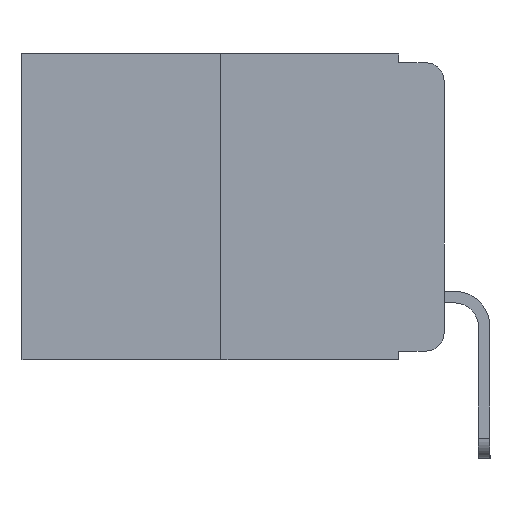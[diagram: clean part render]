
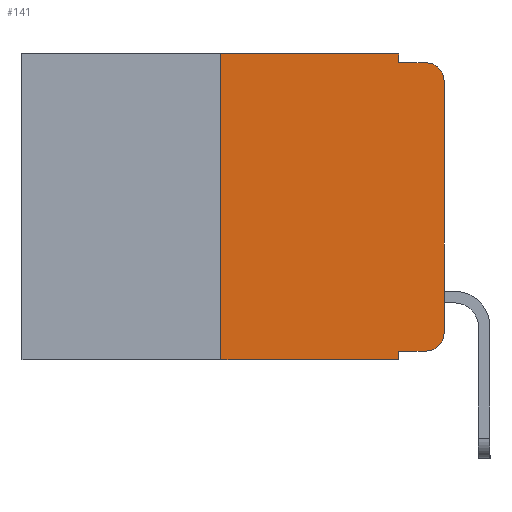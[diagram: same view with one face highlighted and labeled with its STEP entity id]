
A CAD part, left-side view. The second image highlights one B-rep face of the part: STEP entity #141.
In plain terms, the highlighted planar face has unit normal (-1, 0, 0).
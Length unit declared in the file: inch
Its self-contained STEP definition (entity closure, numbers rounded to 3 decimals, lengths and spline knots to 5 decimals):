
#25 = DIRECTION ( 'NONE',  ( 0., 0., 1. ) ) ;
#141 = ADVANCED_FACE ( 'NONE', ( #5684 ), #10027, .F. ) ;
#240 = EDGE_CURVE ( 'NONE', #4264, #10251, #3915, .T. ) ;
#488 = CARTESIAN_POINT ( 'NONE',  ( 0., 0.02, -0.03 ) ) ;
#715 = CARTESIAN_POINT ( 'NONE',  ( 0., 0.02, -0.01 ) ) ;
#745 = DIRECTION ( 'NONE',  ( 0., 0., -1. ) ) ;
#828 = DIRECTION ( 'NONE',  ( -1., 0., 0. ) ) ;
#872 = CARTESIAN_POINT ( 'NONE',  ( 0., 0.051, 0. ) ) ;
#1058 = VECTOR ( 'NONE', #2908, 39.37008 ) ;
#1182 = CARTESIAN_POINT ( 'NONE',  ( 0., 0.02, -0.333 ) ) ;
#1365 = EDGE_CURVE ( 'NONE', #10251, #9961, #12250, .T. ) ;
#1483 = VECTOR ( 'NONE', #25, 39.37008 ) ;
#1521 = VECTOR ( 'NONE', #1560, 39.37008 ) ;
#1560 = DIRECTION ( 'NONE',  ( 0., 0., 1. ) ) ;
#1778 = DIRECTION ( 'NONE',  ( -1., 0., 0. ) ) ;
#1791 = DIRECTION ( 'NONE',  ( 0., -1., 0. ) ) ;
#2551 = ORIENTED_EDGE ( 'NONE', *, *, #5349, .T. ) ;
#2644 = EDGE_CURVE ( 'NONE', #12869, #10065, #5430, .T. ) ;
#2698 = AXIS2_PLACEMENT_3D ( 'NONE', #488, #1778, #5899 ) ;
#2858 = LINE ( 'NONE', #7177, #7730 ) ;
#2908 = DIRECTION ( 'NONE',  ( 0., -1., 0. ) ) ;
#2915 = VERTEX_POINT ( 'NONE', #872 ) ;
#3318 = CARTESIAN_POINT ( 'NONE',  ( 0., 0., 0. ) ) ;
#3397 = EDGE_CURVE ( 'NONE', #5136, #4264, #13299, .T. ) ;
#3454 = ORIENTED_EDGE ( 'NONE', *, *, #7066, .F. ) ;
#3545 = EDGE_LOOP ( 'NONE', ( #9908, #2551, #11814, #5180, #7015, #3454, #7256, #12680, #9693, #5321 ) ) ;
#3559 = LINE ( 'NONE', #4491, #11255 ) ;
#3915 = CIRCLE ( 'NONE', #11914, 0.02 ) ;
#4149 = EDGE_CURVE ( 'NONE', #2915, #12869, #9555, .T. ) ;
#4264 = VERTEX_POINT ( 'NONE', #1182 ) ;
#4368 = CARTESIAN_POINT ( 'NONE',  ( 0., 0.051, -0.343 ) ) ;
#4491 = CARTESIAN_POINT ( 'NONE',  ( 0., 0.051, 0. ) ) ;
#4699 = VECTOR ( 'NONE', #11988, 39.37008 ) ;
#4989 = CIRCLE ( 'NONE', #2698, 0.02 ) ;
#5136 = VERTEX_POINT ( 'NONE', #11007 ) ;
#5180 = ORIENTED_EDGE ( 'NONE', *, *, #4149, .F. ) ;
#5321 = ORIENTED_EDGE ( 'NONE', *, *, #240, .T. ) ;
#5349 = EDGE_CURVE ( 'NONE', #9961, #10065, #4989, .T. ) ;
#5430 = LINE ( 'NONE', #11001, #4699 ) ;
#5605 = DIRECTION ( 'NONE',  ( 0., -1., 0. ) ) ;
#5684 = FACE_OUTER_BOUND ( 'NONE', #3545, .T. ) ;
#5819 = DIRECTION ( 'NONE',  ( 0., 0., -1. ) ) ;
#5899 = DIRECTION ( 'NONE',  ( 0., 0., -1. ) ) ;
#6280 = VERTEX_POINT ( 'NONE', #4368 ) ;
#6712 = VERTEX_POINT ( 'NONE', #10239 ) ;
#7015 = ORIENTED_EDGE ( 'NONE', *, *, #12361, .F. ) ;
#7066 = EDGE_CURVE ( 'NONE', #9452, #6712, #9349, .T. ) ;
#7177 = CARTESIAN_POINT ( 'NONE',  ( 0., 0.473, -0.343 ) ) ;
#7256 = ORIENTED_EDGE ( 'NONE', *, *, #11709, .T. ) ;
#7360 = CARTESIAN_POINT ( 'NONE',  ( 0., 0.051, 0. ) ) ;
#7667 = CARTESIAN_POINT ( 'NONE',  ( 0., 0.051, -0.333 ) ) ;
#7730 = VECTOR ( 'NONE', #1791, 39.37008 ) ;
#7891 = DIRECTION ( 'NONE',  ( 1., 0., 0. ) ) ;
#8069 = EDGE_CURVE ( 'NONE', #5136, #6280, #3559, .T. ) ;
#8197 = VECTOR ( 'NONE', #745, 39.37008 ) ;
#8271 = CARTESIAN_POINT ( 'NONE',  ( 0., 0.25, -0.343 ) ) ;
#8882 = CARTESIAN_POINT ( 'NONE',  ( 0., 0., -0.313 ) ) ;
#8958 = CARTESIAN_POINT ( 'NONE',  ( 0., 0.473, 0. ) ) ;
#9349 = LINE ( 'NONE', #13606, #1521 ) ;
#9452 = VERTEX_POINT ( 'NONE', #8271 ) ;
#9483 = LINE ( 'NONE', #9564, #1058 ) ;
#9555 = LINE ( 'NONE', #7360, #8197 ) ;
#9564 = CARTESIAN_POINT ( 'NONE',  ( 0., 0.473, 0. ) ) ;
#9693 = ORIENTED_EDGE ( 'NONE', *, *, #3397, .T. ) ;
#9908 = ORIENTED_EDGE ( 'NONE', *, *, #1365, .T. ) ;
#9961 = VERTEX_POINT ( 'NONE', #13721 ) ;
#10027 = PLANE ( 'NONE',  #12577 ) ;
#10065 = VERTEX_POINT ( 'NONE', #715 ) ;
#10103 = DIRECTION ( 'NONE',  ( 0., 0., -1. ) ) ;
#10239 = CARTESIAN_POINT ( 'NONE',  ( 0., 0.25, 0. ) ) ;
#10251 = VERTEX_POINT ( 'NONE', #8882 ) ;
#10439 = CARTESIAN_POINT ( 'NONE',  ( 0., 0.02, -0.313 ) ) ;
#11001 = CARTESIAN_POINT ( 'NONE',  ( 0., 0.051, -0.01 ) ) ;
#11007 = CARTESIAN_POINT ( 'NONE',  ( 0., 0.051, -0.333 ) ) ;
#11255 = VECTOR ( 'NONE', #5819, 39.37008 ) ;
#11574 = VECTOR ( 'NONE', #5605, 39.37008 ) ;
#11709 = EDGE_CURVE ( 'NONE', #9452, #6280, #2858, .T. ) ;
#11814 = ORIENTED_EDGE ( 'NONE', *, *, #2644, .F. ) ;
#11914 = AXIS2_PLACEMENT_3D ( 'NONE', #10439, #828, #13827 ) ;
#11988 = DIRECTION ( 'NONE',  ( 0., -1., 0. ) ) ;
#12250 = LINE ( 'NONE', #3318, #1483 ) ;
#12361 = EDGE_CURVE ( 'NONE', #6712, #2915, #9483, .T. ) ;
#12577 = AXIS2_PLACEMENT_3D ( 'NONE', #8958, #7891, #10103 ) ;
#12680 = ORIENTED_EDGE ( 'NONE', *, *, #8069, .F. ) ;
#12869 = VERTEX_POINT ( 'NONE', #14015 ) ;
#13299 = LINE ( 'NONE', #7667, #11574 ) ;
#13606 = CARTESIAN_POINT ( 'NONE',  ( 0., 0.25, 0. ) ) ;
#13721 = CARTESIAN_POINT ( 'NONE',  ( 0., 0., -0.03 ) ) ;
#13827 = DIRECTION ( 'NONE',  ( 0., 0., -1. ) ) ;
#14015 = CARTESIAN_POINT ( 'NONE',  ( 0., 0.051, -0.01 ) ) ;
